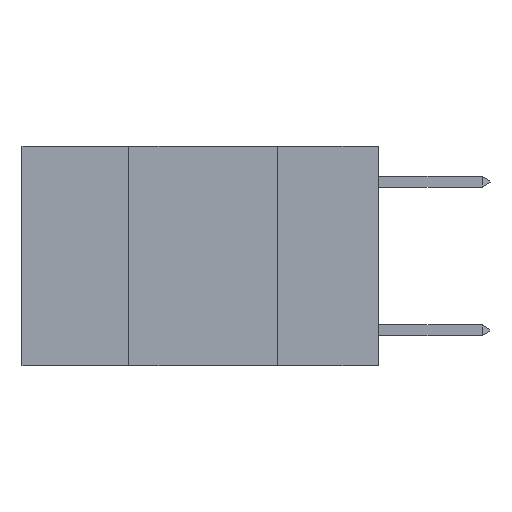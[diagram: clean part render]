
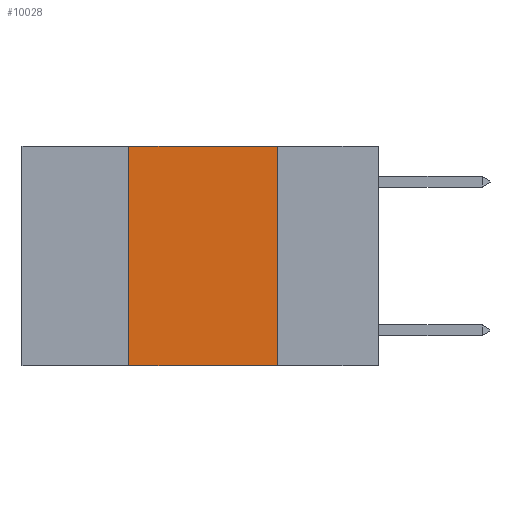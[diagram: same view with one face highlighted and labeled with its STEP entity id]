
A CAD part, left-side view. The second image highlights one B-rep face of the part: STEP entity #10028.
In plain terms, the highlighted planar face has unit normal (-1, 0, 0).
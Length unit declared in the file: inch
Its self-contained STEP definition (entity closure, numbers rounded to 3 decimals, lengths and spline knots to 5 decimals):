
#961 = CARTESIAN_POINT ( 'NONE',  ( 0., 0.17, -0.37 ) ) ;
#1191 = CARTESIAN_POINT ( 'NONE',  ( 0., 0.17, 0. ) ) ;
#1259 = DIRECTION ( 'NONE',  ( 0., 0., -1. ) ) ;
#1519 = VECTOR ( 'NONE', #1259, 39.37008 ) ;
#2540 = ORIENTED_EDGE ( 'NONE', *, *, #19067, .F. ) ;
#2569 = ORIENTED_EDGE ( 'NONE', *, *, #2733, .F. ) ;
#2629 = CARTESIAN_POINT ( 'NONE',  ( 0., 0.6, 0. ) ) ;
#2733 = EDGE_CURVE ( 'NONE', #9601, #15391, #9172, .T. ) ;
#2786 = VERTEX_POINT ( 'NONE', #961 ) ;
#2917 = EDGE_CURVE ( 'NONE', #18874, #2786, #16908, .T. ) ;
#5715 = CARTESIAN_POINT ( 'NONE',  ( 0., 0.42, 0. ) ) ;
#6441 = FACE_OUTER_BOUND ( 'NONE', #12415, .T. ) ;
#6492 = CARTESIAN_POINT ( 'NONE',  ( 0., 0.6, -0.37 ) ) ;
#8228 = VECTOR ( 'NONE', #16475, 39.37008 ) ;
#8390 = EDGE_CURVE ( 'NONE', #18874, #9601, #14139, .T. ) ;
#9172 = LINE ( 'NONE', #2629, #19542 ) ;
#9235 = CARTESIAN_POINT ( 'NONE',  ( 0., 0.42, 0. ) ) ;
#9601 = VERTEX_POINT ( 'NONE', #5715 ) ;
#9906 = LINE ( 'NONE', #15031, #1519 ) ;
#10028 = ADVANCED_FACE ( 'NONE', ( #6441 ), #13009, .F. ) ;
#10217 = ORIENTED_EDGE ( 'NONE', *, *, #2917, .T. ) ;
#11001 = DIRECTION ( 'NONE',  ( 1., 0., 0. ) ) ;
#11117 = CARTESIAN_POINT ( 'NONE',  ( 0., 0.6, 0. ) ) ;
#11334 = DIRECTION ( 'NONE',  ( 0., 0., -1. ) ) ;
#12415 = EDGE_LOOP ( 'NONE', ( #2540, #2569, #14485, #10217 ) ) ;
#12744 = DIRECTION ( 'NONE',  ( 0., -1., 0. ) ) ;
#13009 = PLANE ( 'NONE',  #19989 ) ;
#13207 = VECTOR ( 'NONE', #19289, 39.37008 ) ;
#14139 = LINE ( 'NONE', #9235, #13207 ) ;
#14485 = ORIENTED_EDGE ( 'NONE', *, *, #8390, .F. ) ;
#15031 = CARTESIAN_POINT ( 'NONE',  ( 0., 0.17, 0. ) ) ;
#15391 = VERTEX_POINT ( 'NONE', #1191 ) ;
#16475 = DIRECTION ( 'NONE',  ( 0., -1., 0. ) ) ;
#16908 = LINE ( 'NONE', #6492, #8228 ) ;
#18874 = VERTEX_POINT ( 'NONE', #20995 ) ;
#19067 = EDGE_CURVE ( 'NONE', #15391, #2786, #9906, .T. ) ;
#19289 = DIRECTION ( 'NONE',  ( 0., 0., 1. ) ) ;
#19542 = VECTOR ( 'NONE', #12744, 39.37008 ) ;
#19989 = AXIS2_PLACEMENT_3D ( 'NONE', #11117, #11001, #11334 ) ;
#20995 = CARTESIAN_POINT ( 'NONE',  ( 0., 0.42, -0.37 ) ) ;
